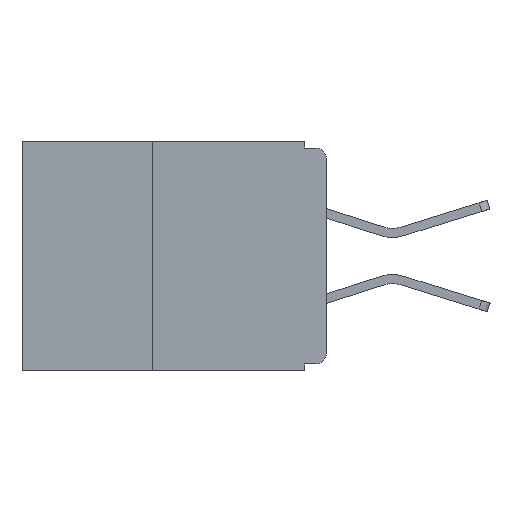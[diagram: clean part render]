
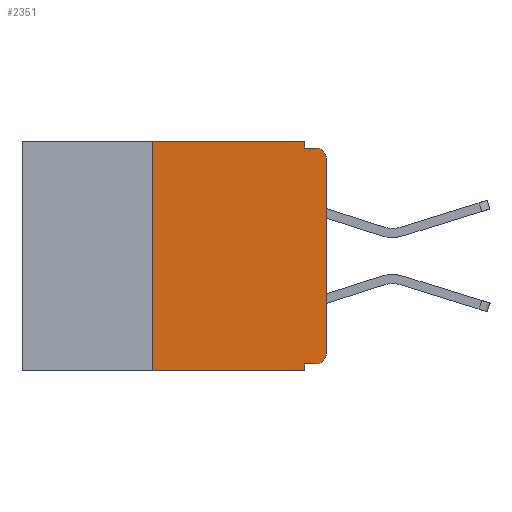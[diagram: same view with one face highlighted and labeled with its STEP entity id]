
A CAD part, left-side view. The second image highlights one B-rep face of the part: STEP entity #2351.
In plain terms, the highlighted planar face has unit normal (-1, 0, 0).
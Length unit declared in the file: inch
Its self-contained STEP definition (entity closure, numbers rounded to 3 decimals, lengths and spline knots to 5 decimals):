
#38 = ORIENTED_EDGE ( 'NONE', *, *, #24872, .T. ) ;
#39 = PLANE ( 'NONE',  #7202 ) ;
#1065 = CARTESIAN_POINT ( 'NONE',  ( 0., 0., -0.305 ) ) ;
#1106 = EDGE_CURVE ( 'NONE', #22253, #15727, #18956, .T. ) ;
#2149 = DIRECTION ( 'NONE',  ( 0., -1., 0. ) ) ;
#2351 = ADVANCED_FACE ( 'NONE', ( #16184 ), #39, .F. ) ;
#2406 = CARTESIAN_POINT ( 'NONE',  ( 0., 0., -0.01 ) ) ;
#2496 = CIRCLE ( 'NONE', #30552, 0.015 ) ;
#4077 = CARTESIAN_POINT ( 'NONE',  ( 0., 0.25, 0. ) ) ;
#4306 = CARTESIAN_POINT ( 'NONE',  ( 0., 0.031, -0.32 ) ) ;
#4440 = CARTESIAN_POINT ( 'NONE',  ( 0., 0.25, -0.33 ) ) ;
#4464 = AXIS2_PLACEMENT_3D ( 'NONE', #21295, #6143, #23808 ) ;
#4505 = VECTOR ( 'NONE', #26003, 39.37008 ) ;
#5454 = VECTOR ( 'NONE', #2149, 39.37008 ) ;
#5470 = DIRECTION ( 'NONE',  ( 0., 0., -1. ) ) ;
#5711 = ORIENTED_EDGE ( 'NONE', *, *, #22259, .F. ) ;
#6143 = DIRECTION ( 'NONE',  ( -1., 0., 0. ) ) ;
#6658 = CARTESIAN_POINT ( 'NONE',  ( 0., 0., -0.32 ) ) ;
#6818 = VERTEX_POINT ( 'NONE', #7287 ) ;
#6959 = LINE ( 'NONE', #20717, #18840 ) ;
#7136 = EDGE_CURVE ( 'NONE', #6818, #15727, #29264, .T. ) ;
#7202 = AXIS2_PLACEMENT_3D ( 'NONE', #32144, #31514, #31966 ) ;
#7287 = CARTESIAN_POINT ( 'NONE',  ( 0., 0., -0.025 ) ) ;
#7973 = LINE ( 'NONE', #19557, #32347 ) ;
#8093 = ORIENTED_EDGE ( 'NONE', *, *, #7136, .T. ) ;
#8295 = ORIENTED_EDGE ( 'NONE', *, *, #21278, .T. ) ;
#8773 = EDGE_CURVE ( 'NONE', #25861, #22556, #19703, .T. ) ;
#9237 = DIRECTION ( 'NONE',  ( 0., 1., 0. ) ) ;
#9301 = VECTOR ( 'NONE', #9237, 39.37008 ) ;
#10058 = EDGE_CURVE ( 'NONE', #12819, #18179, #2496, .T. ) ;
#10156 = EDGE_CURVE ( 'NONE', #14671, #28049, #6959, .T. ) ;
#10290 = DIRECTION ( 'NONE',  ( -1., 0., 0. ) ) ;
#10481 = CARTESIAN_POINT ( 'NONE',  ( 0., 0.25, -0.33 ) ) ;
#10920 = CARTESIAN_POINT ( 'NONE',  ( 0., 0.015, -0.01 ) ) ;
#10945 = EDGE_CURVE ( 'NONE', #12819, #14671, #29401, .T. ) ;
#12150 = DIRECTION ( 'NONE',  ( 0., -1., 0. ) ) ;
#12819 = VERTEX_POINT ( 'NONE', #31878 ) ;
#12896 = ORIENTED_EDGE ( 'NONE', *, *, #10058, .T. ) ;
#13026 = CARTESIAN_POINT ( 'NONE',  ( 0., 0.031, 0. ) ) ;
#13077 = VECTOR ( 'NONE', #28084, 39.37008 ) ;
#13382 = LINE ( 'NONE', #31350, #19235 ) ;
#14671 = VERTEX_POINT ( 'NONE', #4306 ) ;
#15342 = ORIENTED_EDGE ( 'NONE', *, *, #18698, .F. ) ;
#15727 = VERTEX_POINT ( 'NONE', #10920 ) ;
#15755 = VERTEX_POINT ( 'NONE', #21007 ) ;
#15829 = DIRECTION ( 'NONE',  ( 0., 0., -1. ) ) ;
#15990 = ORIENTED_EDGE ( 'NONE', *, *, #10156, .F. ) ;
#16184 = FACE_OUTER_BOUND ( 'NONE', #27956, .T. ) ;
#18074 = LINE ( 'NONE', #23455, #4505 ) ;
#18179 = VERTEX_POINT ( 'NONE', #1065 ) ;
#18698 = EDGE_CURVE ( 'NONE', #22556, #15755, #18074, .T. ) ;
#18840 = VECTOR ( 'NONE', #15829, 39.37008 ) ;
#18857 = DIRECTION ( 'NONE',  ( 0., 0., 1. ) ) ;
#18956 = LINE ( 'NONE', #2406, #5454 ) ;
#19235 = VECTOR ( 'NONE', #18857, 39.37008 ) ;
#19557 = CARTESIAN_POINT ( 'NONE',  ( 0., 0.437, -0.33 ) ) ;
#19703 = LINE ( 'NONE', #10481, #13077 ) ;
#20717 = CARTESIAN_POINT ( 'NONE',  ( 0., 0.031, -0.33 ) ) ;
#21007 = CARTESIAN_POINT ( 'NONE',  ( 0., 0.031, 0. ) ) ;
#21278 = EDGE_CURVE ( 'NONE', #25861, #28049, #7973, .T. ) ;
#21295 = CARTESIAN_POINT ( 'NONE',  ( 0., 0.015, -0.025 ) ) ;
#21477 = ORIENTED_EDGE ( 'NONE', *, *, #10945, .F. ) ;
#22253 = VERTEX_POINT ( 'NONE', #28155 ) ;
#22259 = EDGE_CURVE ( 'NONE', #15755, #22253, #24856, .T. ) ;
#22556 = VERTEX_POINT ( 'NONE', #4077 ) ;
#22642 = CARTESIAN_POINT ( 'NONE',  ( 0., 0.031, -0.33 ) ) ;
#23455 = CARTESIAN_POINT ( 'NONE',  ( 0., 0.437, 0. ) ) ;
#23808 = DIRECTION ( 'NONE',  ( 0., 0., -1. ) ) ;
#24067 = VECTOR ( 'NONE', #5470, 39.37008 ) ;
#24856 = LINE ( 'NONE', #13026, #24067 ) ;
#24872 = EDGE_CURVE ( 'NONE', #18179, #6818, #13382, .T. ) ;
#25325 = CARTESIAN_POINT ( 'NONE',  ( 0., 0.015, -0.305 ) ) ;
#25861 = VERTEX_POINT ( 'NONE', #4440 ) ;
#26003 = DIRECTION ( 'NONE',  ( 0., -1., 0. ) ) ;
#27890 = DIRECTION ( 'NONE',  ( 0., 0., -1. ) ) ;
#27956 = EDGE_LOOP ( 'NONE', ( #38, #8093, #29695, #5711, #15342, #29468, #8295, #15990, #21477, #12896 ) ) ;
#28049 = VERTEX_POINT ( 'NONE', #22642 ) ;
#28084 = DIRECTION ( 'NONE',  ( 0., 0., 1. ) ) ;
#28155 = CARTESIAN_POINT ( 'NONE',  ( 0., 0.031, -0.01 ) ) ;
#29264 = CIRCLE ( 'NONE', #4464, 0.015 ) ;
#29401 = LINE ( 'NONE', #6658, #9301 ) ;
#29468 = ORIENTED_EDGE ( 'NONE', *, *, #8773, .F. ) ;
#29695 = ORIENTED_EDGE ( 'NONE', *, *, #1106, .F. ) ;
#30552 = AXIS2_PLACEMENT_3D ( 'NONE', #25325, #10290, #27890 ) ;
#31350 = CARTESIAN_POINT ( 'NONE',  ( 0., 0., 0. ) ) ;
#31514 = DIRECTION ( 'NONE',  ( 1., 0., 0. ) ) ;
#31878 = CARTESIAN_POINT ( 'NONE',  ( 0., 0.015, -0.32 ) ) ;
#31966 = DIRECTION ( 'NONE',  ( 0., 0., -1. ) ) ;
#32144 = CARTESIAN_POINT ( 'NONE',  ( 0., 0.437, 0. ) ) ;
#32347 = VECTOR ( 'NONE', #12150, 39.37008 ) ;
